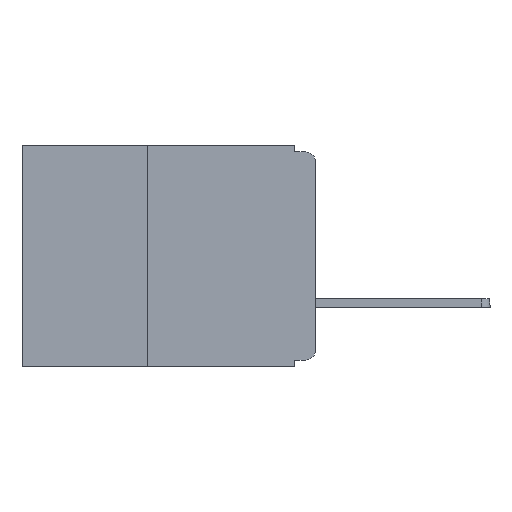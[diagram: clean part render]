
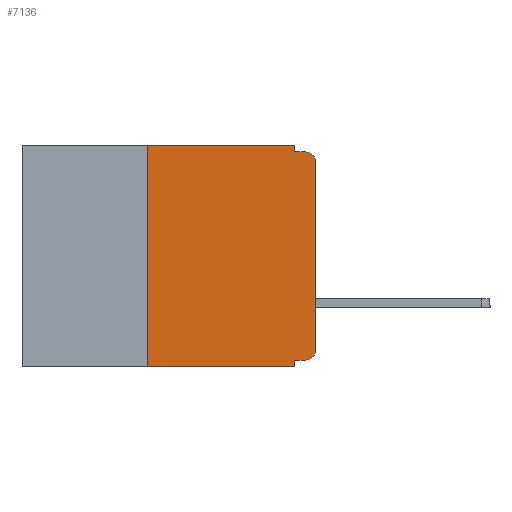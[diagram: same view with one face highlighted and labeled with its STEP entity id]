
A CAD part, left-side view. The second image highlights one B-rep face of the part: STEP entity #7136.
In plain terms, the highlighted planar face has unit normal (-1, 0, 0).
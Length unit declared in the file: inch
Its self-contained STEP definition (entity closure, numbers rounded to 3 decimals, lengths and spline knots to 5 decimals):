
#206 = DIRECTION ( 'NONE',  ( 0., 0., 1. ) ) ;
#322 = CARTESIAN_POINT ( 'NONE',  ( 0., 0.25, -0.33 ) ) ;
#654 = VERTEX_POINT ( 'NONE', #2388 ) ;
#937 = ORIENTED_EDGE ( 'NONE', *, *, #14971, .F. ) ;
#1219 = LINE ( 'NONE', #31565, #21280 ) ;
#1404 = CARTESIAN_POINT ( 'NONE',  ( 0., 0.25, 0. ) ) ;
#1592 = EDGE_CURVE ( 'NONE', #654, #14968, #21927, .T. ) ;
#1617 = CARTESIAN_POINT ( 'NONE',  ( 0., 0.015, -0.01 ) ) ;
#2000 = VERTEX_POINT ( 'NONE', #1617 ) ;
#2048 = EDGE_CURVE ( 'NONE', #13107, #32180, #21888, .T. ) ;
#2388 = CARTESIAN_POINT ( 'NONE',  ( 0., 0.015, -0.32 ) ) ;
#2810 = CARTESIAN_POINT ( 'NONE',  ( 0., 0.437, 0. ) ) ;
#3115 = CARTESIAN_POINT ( 'NONE',  ( 0., 0., -0.305 ) ) ;
#4049 = EDGE_CURVE ( 'NONE', #654, #30640, #19294, .T. ) ;
#5104 = CARTESIAN_POINT ( 'NONE',  ( 0., 0.031, 0. ) ) ;
#5358 = ORIENTED_EDGE ( 'NONE', *, *, #25456, .T. ) ;
#5415 = CARTESIAN_POINT ( 'NONE',  ( 0., 0.031, -0.32 ) ) ;
#5436 = DIRECTION ( 'NONE',  ( 1., 0., 0. ) ) ;
#5657 = EDGE_LOOP ( 'NONE', ( #13954, #5358, #14821, #12610, #8929, #26075, #6922, #937, #10320, #14480 ) ) ;
#5739 = CARTESIAN_POINT ( 'NONE',  ( 0., 0.437, -0.33 ) ) ;
#6218 = VECTOR ( 'NONE', #9870, 39.37008 ) ;
#6366 = CARTESIAN_POINT ( 'NONE',  ( 0., 0.031, -0.01 ) ) ;
#6533 = CARTESIAN_POINT ( 'NONE',  ( 0., 0., 0. ) ) ;
#6922 = ORIENTED_EDGE ( 'NONE', *, *, #16803, .T. ) ;
#6994 = VECTOR ( 'NONE', #31992, 39.37008 ) ;
#7136 = ADVANCED_FACE ( 'NONE', ( #17102 ), #31572, .F. ) ;
#8305 = CARTESIAN_POINT ( 'NONE',  ( 0., 0.031, 0. ) ) ;
#8386 = DIRECTION ( 'NONE',  ( 0., -1., 0. ) ) ;
#8929 = ORIENTED_EDGE ( 'NONE', *, *, #13673, .F. ) ;
#9870 = DIRECTION ( 'NONE',  ( 0., 1., 0. ) ) ;
#10320 = ORIENTED_EDGE ( 'NONE', *, *, #4049, .F. ) ;
#10515 = DIRECTION ( 'NONE',  ( 0., 0., -1. ) ) ;
#10719 = DIRECTION ( 'NONE',  ( 0., 0., -1. ) ) ;
#10754 = DIRECTION ( 'NONE',  ( -1., 0., 0. ) ) ;
#10759 = CARTESIAN_POINT ( 'NONE',  ( 0., 0.015, -0.305 ) ) ;
#10805 = DIRECTION ( 'NONE',  ( -1., 0., 0. ) ) ;
#11170 = EDGE_CURVE ( 'NONE', #24464, #2000, #1219, .T. ) ;
#12001 = AXIS2_PLACEMENT_3D ( 'NONE', #2810, #5436, #23826 ) ;
#12610 = ORIENTED_EDGE ( 'NONE', *, *, #16081, .F. ) ;
#12695 = VECTOR ( 'NONE', #8386, 39.37008 ) ;
#13107 = VERTEX_POINT ( 'NONE', #33569 ) ;
#13384 = DIRECTION ( 'NONE',  ( 0., -1., 0. ) ) ;
#13673 = EDGE_CURVE ( 'NONE', #32180, #21253, #15743, .T. ) ;
#13954 = ORIENTED_EDGE ( 'NONE', *, *, #15149, .T. ) ;
#13997 = LINE ( 'NONE', #16214, #6994 ) ;
#14480 = ORIENTED_EDGE ( 'NONE', *, *, #1592, .T. ) ;
#14821 = ORIENTED_EDGE ( 'NONE', *, *, #11170, .F. ) ;
#14968 = VERTEX_POINT ( 'NONE', #3115 ) ;
#14971 = EDGE_CURVE ( 'NONE', #30640, #16254, #13997, .T. ) ;
#15149 = EDGE_CURVE ( 'NONE', #14968, #17095, #23010, .T. ) ;
#15743 = LINE ( 'NONE', #30551, #28873 ) ;
#16081 = EDGE_CURVE ( 'NONE', #21253, #24464, #22087, .T. ) ;
#16214 = CARTESIAN_POINT ( 'NONE',  ( 0., 0.031, -0.33 ) ) ;
#16254 = VERTEX_POINT ( 'NONE', #32027 ) ;
#16803 = EDGE_CURVE ( 'NONE', #13107, #16254, #33579, .T. ) ;
#16974 = DIRECTION ( 'NONE',  ( 0., 0., 1. ) ) ;
#17095 = VERTEX_POINT ( 'NONE', #28343 ) ;
#17102 = FACE_OUTER_BOUND ( 'NONE', #5657, .T. ) ;
#19294 = LINE ( 'NONE', #25557, #6218 ) ;
#21057 = VECTOR ( 'NONE', #206, 39.37008 ) ;
#21253 = VERTEX_POINT ( 'NONE', #8305 ) ;
#21280 = VECTOR ( 'NONE', #13384, 39.37008 ) ;
#21592 = AXIS2_PLACEMENT_3D ( 'NONE', #26498, #10805, #29146 ) ;
#21888 = LINE ( 'NONE', #322, #21057 ) ;
#21927 = CIRCLE ( 'NONE', #33610, 0.015 ) ;
#22087 = LINE ( 'NONE', #5104, #22943 ) ;
#22782 = DIRECTION ( 'NONE',  ( 0., -1., 0. ) ) ;
#22943 = VECTOR ( 'NONE', #10515, 39.37008 ) ;
#23010 = LINE ( 'NONE', #6533, #29965 ) ;
#23826 = DIRECTION ( 'NONE',  ( 0., 0., -1. ) ) ;
#24464 = VERTEX_POINT ( 'NONE', #6366 ) ;
#25456 = EDGE_CURVE ( 'NONE', #17095, #2000, #29921, .T. ) ;
#25557 = CARTESIAN_POINT ( 'NONE',  ( 0., 0., -0.32 ) ) ;
#26075 = ORIENTED_EDGE ( 'NONE', *, *, #2048, .F. ) ;
#26498 = CARTESIAN_POINT ( 'NONE',  ( 0., 0.015, -0.025 ) ) ;
#28343 = CARTESIAN_POINT ( 'NONE',  ( 0., 0., -0.025 ) ) ;
#28873 = VECTOR ( 'NONE', #22782, 39.37008 ) ;
#29146 = DIRECTION ( 'NONE',  ( 0., 0., -1. ) ) ;
#29921 = CIRCLE ( 'NONE', #21592, 0.015 ) ;
#29965 = VECTOR ( 'NONE', #16974, 39.37008 ) ;
#30551 = CARTESIAN_POINT ( 'NONE',  ( 0., 0.437, 0. ) ) ;
#30640 = VERTEX_POINT ( 'NONE', #5415 ) ;
#31565 = CARTESIAN_POINT ( 'NONE',  ( 0., 0., -0.01 ) ) ;
#31572 = PLANE ( 'NONE',  #12001 ) ;
#31992 = DIRECTION ( 'NONE',  ( 0., 0., -1. ) ) ;
#32027 = CARTESIAN_POINT ( 'NONE',  ( 0., 0.031, -0.33 ) ) ;
#32180 = VERTEX_POINT ( 'NONE', #1404 ) ;
#33569 = CARTESIAN_POINT ( 'NONE',  ( 0., 0.25, -0.33 ) ) ;
#33579 = LINE ( 'NONE', #5739, #12695 ) ;
#33610 = AXIS2_PLACEMENT_3D ( 'NONE', #10759, #10754, #10719 ) ;
